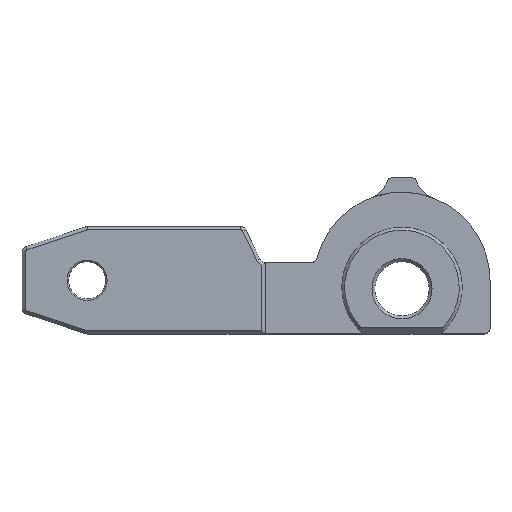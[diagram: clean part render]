
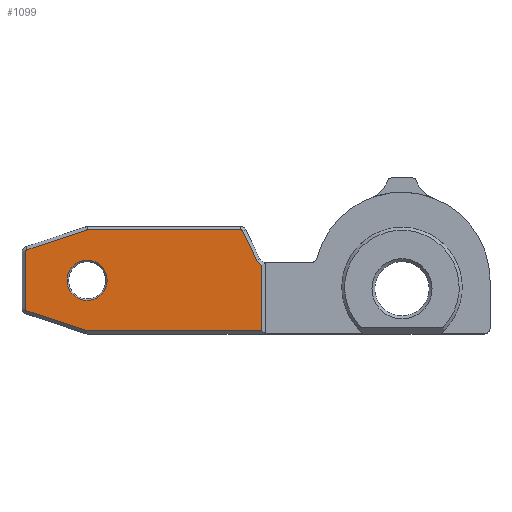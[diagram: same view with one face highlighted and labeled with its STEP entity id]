
A CAD part, top view. The second image highlights one B-rep face of the part: STEP entity #1099.
In plain terms, the highlighted planar face has unit normal (0, 0, 1).
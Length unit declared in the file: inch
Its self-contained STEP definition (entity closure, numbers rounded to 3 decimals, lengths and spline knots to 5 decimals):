
#36=FACE_BOUND('',#364,.T.);
#76=LINE('',#1800,#173);
#77=LINE('',#1802,#174);
#78=LINE('',#1806,#175);
#79=LINE('',#1810,#176);
#80=LINE('',#1814,#177);
#81=LINE('',#1818,#178);
#82=LINE('',#1822,#179);
#173=VECTOR('',#1441,0.3937);
#174=VECTOR('',#1442,0.3937);
#175=VECTOR('',#1445,0.3937);
#176=VECTOR('',#1448,0.3937);
#177=VECTOR('',#1451,0.3937);
#178=VECTOR('',#1454,0.3937);
#179=VECTOR('',#1457,0.3937);
#243=PLANE('',#1217);
#291=FACE_OUTER_BOUND('',#363,.T.);
#363=EDGE_LOOP('',(#848,#849,#850,#851,#852,#853,#854,#855,#856,#857,#858,
#859,#860));
#364=EDGE_LOOP('',(#861));
#440=CIRCLE('',#1216,0.07);
#441=CIRCLE('',#1218,0.0315);
#442=CIRCLE('',#1219,0.0085);
#443=CIRCLE('',#1220,0.0085);
#444=CIRCLE('',#1221,0.0085);
#445=CIRCLE('',#1222,0.0085);
#446=CIRCLE('',#1223,0.0085);
#525=VERTEX_POINT('',#1794);
#526=VERTEX_POINT('',#1798);
#527=VERTEX_POINT('',#1799);
#528=VERTEX_POINT('',#1801);
#529=VERTEX_POINT('',#1803);
#530=VERTEX_POINT('',#1805);
#531=VERTEX_POINT('',#1807);
#532=VERTEX_POINT('',#1809);
#533=VERTEX_POINT('',#1811);
#534=VERTEX_POINT('',#1813);
#535=VERTEX_POINT('',#1815);
#536=VERTEX_POINT('',#1817);
#537=VERTEX_POINT('',#1819);
#538=VERTEX_POINT('',#1821);
#642=EDGE_CURVE('',#525,#525,#440,.T.);
#644=EDGE_CURVE('',#526,#527,#76,.T.);
#645=EDGE_CURVE('',#528,#526,#77,.T.);
#646=EDGE_CURVE('',#529,#528,#441,.T.);
#647=EDGE_CURVE('',#530,#529,#78,.T.);
#648=EDGE_CURVE('',#531,#530,#442,.T.);
#649=EDGE_CURVE('',#532,#531,#79,.T.);
#650=EDGE_CURVE('',#533,#532,#443,.T.);
#651=EDGE_CURVE('',#534,#533,#80,.T.);
#652=EDGE_CURVE('',#535,#534,#444,.T.);
#653=EDGE_CURVE('',#536,#535,#81,.T.);
#654=EDGE_CURVE('',#537,#536,#445,.T.);
#655=EDGE_CURVE('',#538,#537,#82,.T.);
#656=EDGE_CURVE('',#527,#538,#446,.T.);
#848=ORIENTED_EDGE('',*,*,#644,.F.);
#849=ORIENTED_EDGE('',*,*,#645,.F.);
#850=ORIENTED_EDGE('',*,*,#646,.F.);
#851=ORIENTED_EDGE('',*,*,#647,.F.);
#852=ORIENTED_EDGE('',*,*,#648,.F.);
#853=ORIENTED_EDGE('',*,*,#649,.F.);
#854=ORIENTED_EDGE('',*,*,#650,.F.);
#855=ORIENTED_EDGE('',*,*,#651,.F.);
#856=ORIENTED_EDGE('',*,*,#652,.F.);
#857=ORIENTED_EDGE('',*,*,#653,.F.);
#858=ORIENTED_EDGE('',*,*,#654,.F.);
#859=ORIENTED_EDGE('',*,*,#655,.F.);
#860=ORIENTED_EDGE('',*,*,#656,.F.);
#861=ORIENTED_EDGE('',*,*,#642,.F.);
#1099=ADVANCED_FACE('',(#291,#36),#243,.T.);
#1216=AXIS2_PLACEMENT_3D('',#1795,#1436,#1437);
#1217=AXIS2_PLACEMENT_3D('',#1797,#1439,#1440);
#1218=AXIS2_PLACEMENT_3D('',#1804,#1443,#1444);
#1219=AXIS2_PLACEMENT_3D('',#1808,#1446,#1447);
#1220=AXIS2_PLACEMENT_3D('',#1812,#1449,#1450);
#1221=AXIS2_PLACEMENT_3D('',#1816,#1452,#1453);
#1222=AXIS2_PLACEMENT_3D('',#1820,#1455,#1456);
#1223=AXIS2_PLACEMENT_3D('',#1823,#1458,#1459);
#1436=DIRECTION('center_axis',(0.,0.,1.));
#1437=DIRECTION('ref_axis',(-1.,0.,0.));
#1439=DIRECTION('center_axis',(0.,0.,1.));
#1440=DIRECTION('ref_axis',(1.,0.,0.));
#1441=DIRECTION('',(-1.,0.,0.));
#1442=DIRECTION('',(0.,-1.,0.));
#1443=DIRECTION('center_axis',(0.,0.,1.));
#1444=DIRECTION('ref_axis',(-0.533,-0.846,0.));
#1445=DIRECTION('',(0.433,-0.902,0.));
#1446=DIRECTION('center_axis',(0.,0.,-1.));
#1447=DIRECTION('ref_axis',(0.533,0.846,0.));
#1448=DIRECTION('',(1.,0.,0.));
#1449=DIRECTION('center_axis',(0.,0.,-1.));
#1450=DIRECTION('ref_axis',(-0.16,0.987,0.));
#1451=DIRECTION('',(0.949,0.316,0.));
#1452=DIRECTION('center_axis',(0.,0.,-1.));
#1453=DIRECTION('ref_axis',(-0.811,0.585,0.));
#1454=DIRECTION('',(0.,1.,0.));
#1455=DIRECTION('center_axis',(0.,0.,-1.));
#1456=DIRECTION('ref_axis',(-0.811,-0.585,0.));
#1457=DIRECTION('',(-0.949,0.316,0.));
#1458=DIRECTION('center_axis',(0.,0.,-1.));
#1459=DIRECTION('ref_axis',(-0.16,-0.987,0.));
#1794=CARTESIAN_POINT('',(-1.03,-0.085,0.1365));
#1795=CARTESIAN_POINT('Origin',(-1.1,-0.085,0.1365));
#1797=CARTESIAN_POINT('Origin',(0.,0.,0.1365));
#1798=CARTESIAN_POINT('',(-0.48944,-0.261,0.1365));
#1799=CARTESIAN_POINT('',(-1.09925,-0.261,0.1365));
#1800=CARTESIAN_POINT('',(-0.66375,-0.261,0.1365));
#1801=CARTESIAN_POINT('',(-0.48944,-0.03204,0.1365));
#1802=CARTESIAN_POINT('',(-0.48944,-0.07375,0.1365));
#1803=CARTESIAN_POINT('',(-0.50689,-0.01613,0.1365));
#1804=CARTESIAN_POINT('Origin',(-0.4785,-0.0025,
0.1365));
#1805=CARTESIAN_POINT('',(-0.556,0.08618,0.1365));
#1806=CARTESIAN_POINT('',(-0.47486,-0.08287,0.1365));
#1807=CARTESIAN_POINT('',(-0.56367,0.091,0.1365));
#1808=CARTESIAN_POINT('Origin',(-0.56367,0.0825,0.1365));
#1809=CARTESIAN_POINT('',(-1.09925,0.091,0.1365));
#1810=CARTESIAN_POINT('',(-0.24554,0.091,0.1365));
#1811=CARTESIAN_POINT('',(-1.10194,0.09056,0.1365));
#1812=CARTESIAN_POINT('Origin',(-1.09925,0.0825,0.1365));
#1813=CARTESIAN_POINT('',(-1.31019,0.02115,0.1365));
#1814=CARTESIAN_POINT('',(-0.67436,0.23309,0.1365));
#1815=CARTESIAN_POINT('',(-1.316,0.01308,0.1365));
#1816=CARTESIAN_POINT('Origin',(-1.3075,0.01308,0.1365));
#1817=CARTESIAN_POINT('',(-1.316,-0.18308,0.1365));
#1818=CARTESIAN_POINT('',(-1.316,0.05125,0.1365));
#1819=CARTESIAN_POINT('',(-1.31019,-0.19115,0.1365));
#1820=CARTESIAN_POINT('Origin',(-1.3075,-0.18308,0.1365));
#1821=CARTESIAN_POINT('',(-1.10194,-0.26056,0.1365));
#1822=CARTESIAN_POINT('',(-0.69986,-0.39459,0.1365));
#1823=CARTESIAN_POINT('Origin',(-1.09925,-0.2525,0.1365));
